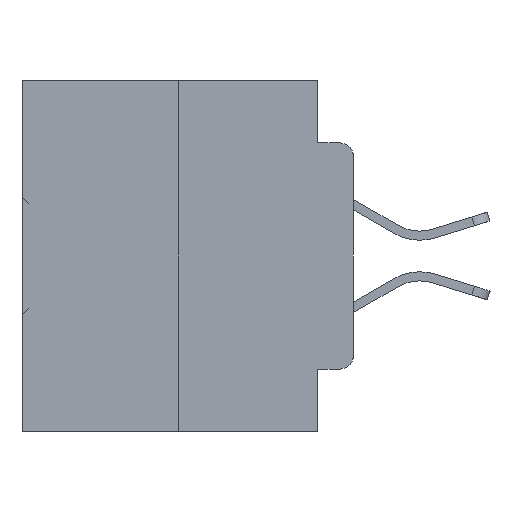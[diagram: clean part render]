
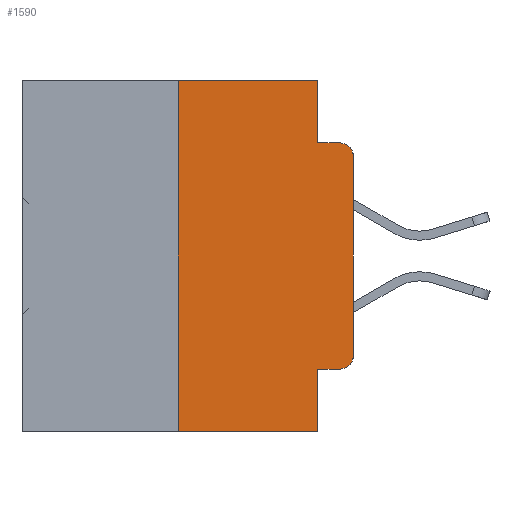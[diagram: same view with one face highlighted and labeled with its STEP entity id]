
A CAD part, left-side view. The second image highlights one B-rep face of the part: STEP entity #1590.
In plain terms, the highlighted planar face has unit normal (-1, 0, 0).
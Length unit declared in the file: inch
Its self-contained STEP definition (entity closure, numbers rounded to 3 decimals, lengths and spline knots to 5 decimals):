
#849 = CARTESIAN_POINT ( 'NONE',  ( 0., 0.02, -0.4115 ) ) ;
#1235 = LINE ( 'NONE', #35393, #11117 ) ;
#1590 = ADVANCED_FACE ( 'NONE', ( #17342 ), #5550, .F. ) ;
#2714 = LINE ( 'NONE', #26049, #8044 ) ;
#4471 = CARTESIAN_POINT ( 'NONE',  ( 0., 0.25, -0.5 ) ) ;
#4784 = CARTESIAN_POINT ( 'NONE',  ( 0., 0.051, 0. ) ) ;
#4854 = EDGE_CURVE ( 'NONE', #24639, #13450, #2714, .T. ) ;
#5306 = AXIS2_PLACEMENT_3D ( 'NONE', #25701, #11436, #6289 ) ;
#5316 = CARTESIAN_POINT ( 'NONE',  ( 0., 0., -0.3915 ) ) ;
#5348 = DIRECTION ( 'NONE',  ( 0., 0., -1. ) ) ;
#5550 = PLANE ( 'NONE',  #5306 ) ;
#6289 = DIRECTION ( 'NONE',  ( 0., 0., -1. ) ) ;
#6472 = ORIENTED_EDGE ( 'NONE', *, *, #21954, .F. ) ;
#7956 = DIRECTION ( 'NONE',  ( 0., 0., -1. ) ) ;
#8044 = VECTOR ( 'NONE', #14275, 39.37008 ) ;
#8577 = CARTESIAN_POINT ( 'NONE',  ( 0., 0.051, 0. ) ) ;
#8729 = ORIENTED_EDGE ( 'NONE', *, *, #13873, .F. ) ;
#8982 = CARTESIAN_POINT ( 'NONE',  ( 0., 0.051, -0.0885 ) ) ;
#9160 = LINE ( 'NONE', #8982, #25146 ) ;
#9409 = CARTESIAN_POINT ( 'NONE',  ( 0., 0.051, -0.4115 ) ) ;
#9589 = ORIENTED_EDGE ( 'NONE', *, *, #22136, .T. ) ;
#9654 = EDGE_CURVE ( 'NONE', #20656, #35957, #35000, .T. ) ;
#9702 = VERTEX_POINT ( 'NONE', #5316 ) ;
#11117 = VECTOR ( 'NONE', #29701, 39.37008 ) ;
#11376 = VECTOR ( 'NONE', #5348, 39.37008 ) ;
#11436 = DIRECTION ( 'NONE',  ( 1., 0., 0. ) ) ;
#11854 = ORIENTED_EDGE ( 'NONE', *, *, #24935, .F. ) ;
#12412 = ORIENTED_EDGE ( 'NONE', *, *, #24043, .T. ) ;
#12567 = CARTESIAN_POINT ( 'NONE',  ( 0., 0.473, 0. ) ) ;
#12810 = CARTESIAN_POINT ( 'NONE',  ( 0., 0.02, -0.0885 ) ) ;
#13204 = VERTEX_POINT ( 'NONE', #9409 ) ;
#13450 = VERTEX_POINT ( 'NONE', #31621 ) ;
#13873 = EDGE_CURVE ( 'NONE', #13204, #13450, #14097, .T. ) ;
#14097 = LINE ( 'NONE', #8577, #21245 ) ;
#14275 = DIRECTION ( 'NONE',  ( 0., -1., 0. ) ) ;
#14975 = LINE ( 'NONE', #20490, #28201 ) ;
#16247 = AXIS2_PLACEMENT_3D ( 'NONE', #16725, #24890, #7956 ) ;
#16725 = CARTESIAN_POINT ( 'NONE',  ( 0., 0.02, -0.1085 ) ) ;
#17342 = FACE_OUTER_BOUND ( 'NONE', #27610, .T. ) ;
#19025 = LINE ( 'NONE', #12567, #22016 ) ;
#19763 = ORIENTED_EDGE ( 'NONE', *, *, #33276, .F. ) ;
#19783 = LINE ( 'NONE', #23009, #11376 ) ;
#19820 = CARTESIAN_POINT ( 'NONE',  ( 0., 0.051, -0.0885 ) ) ;
#20213 = DIRECTION ( 'NONE',  ( -1., 0., 0. ) ) ;
#20371 = DIRECTION ( 'NONE',  ( 0., 0., -1. ) ) ;
#20401 = CARTESIAN_POINT ( 'NONE',  ( 0., 0.02, -0.3915 ) ) ;
#20490 = CARTESIAN_POINT ( 'NONE',  ( 0., 0., 0. ) ) ;
#20656 = VERTEX_POINT ( 'NONE', #30161 ) ;
#20673 = CARTESIAN_POINT ( 'NONE',  ( 0., 0.25, 0. ) ) ;
#21245 = VECTOR ( 'NONE', #20371, 39.37008 ) ;
#21954 = EDGE_CURVE ( 'NONE', #34160, #22125, #19025, .T. ) ;
#22016 = VECTOR ( 'NONE', #30053, 39.37008 ) ;
#22125 = VERTEX_POINT ( 'NONE', #4784 ) ;
#22136 = EDGE_CURVE ( 'NONE', #13204, #25064, #34033, .T. ) ;
#22155 = ORIENTED_EDGE ( 'NONE', *, *, #24896, .T. ) ;
#22590 = ORIENTED_EDGE ( 'NONE', *, *, #27533, .F. ) ;
#23009 = CARTESIAN_POINT ( 'NONE',  ( 0., 0.051, 0. ) ) ;
#23064 = DIRECTION ( 'NONE',  ( 0., 0., -1. ) ) ;
#24043 = EDGE_CURVE ( 'NONE', #9702, #20656, #14975, .T. ) ;
#24639 = VERTEX_POINT ( 'NONE', #4471 ) ;
#24890 = DIRECTION ( 'NONE',  ( -1., 0., 0. ) ) ;
#24896 = EDGE_CURVE ( 'NONE', #25064, #9702, #26356, .T. ) ;
#24935 = EDGE_CURVE ( 'NONE', #27840, #35957, #9160, .T. ) ;
#24988 = ORIENTED_EDGE ( 'NONE', *, *, #4854, .T. ) ;
#25064 = VERTEX_POINT ( 'NONE', #849 ) ;
#25146 = VECTOR ( 'NONE', #34459, 39.37008 ) ;
#25701 = CARTESIAN_POINT ( 'NONE',  ( 0., 0.473, 0. ) ) ;
#26049 = CARTESIAN_POINT ( 'NONE',  ( 0., 0.473, -0.5 ) ) ;
#26356 = CIRCLE ( 'NONE', #32386, 0.02 ) ;
#27533 = EDGE_CURVE ( 'NONE', #24639, #34160, #1235, .T. ) ;
#27610 = EDGE_LOOP ( 'NONE', ( #12412, #32793, #11854, #19763, #6472, #22590, #24988, #8729, #9589, #22155 ) ) ;
#27840 = VERTEX_POINT ( 'NONE', #19820 ) ;
#28201 = VECTOR ( 'NONE', #32445, 39.37008 ) ;
#29701 = DIRECTION ( 'NONE',  ( 0., 0., 1. ) ) ;
#30053 = DIRECTION ( 'NONE',  ( 0., -1., 0. ) ) ;
#30161 = CARTESIAN_POINT ( 'NONE',  ( 0., 0., -0.1085 ) ) ;
#30804 = CARTESIAN_POINT ( 'NONE',  ( 0., 0.051, -0.4115 ) ) ;
#31621 = CARTESIAN_POINT ( 'NONE',  ( 0., 0.051, -0.5 ) ) ;
#32386 = AXIS2_PLACEMENT_3D ( 'NONE', #20401, #20213, #23064 ) ;
#32445 = DIRECTION ( 'NONE',  ( 0., 0., 1. ) ) ;
#32793 = ORIENTED_EDGE ( 'NONE', *, *, #9654, .T. ) ;
#33276 = EDGE_CURVE ( 'NONE', #22125, #27840, #19783, .T. ) ;
#33521 = VECTOR ( 'NONE', #36685, 39.37008 ) ;
#34033 = LINE ( 'NONE', #30804, #33521 ) ;
#34160 = VERTEX_POINT ( 'NONE', #20673 ) ;
#34459 = DIRECTION ( 'NONE',  ( 0., -1., 0. ) ) ;
#35000 = CIRCLE ( 'NONE', #16247, 0.02 ) ;
#35393 = CARTESIAN_POINT ( 'NONE',  ( 0., 0.25, 0. ) ) ;
#35957 = VERTEX_POINT ( 'NONE', #12810 ) ;
#36685 = DIRECTION ( 'NONE',  ( 0., -1., 0. ) ) ;
